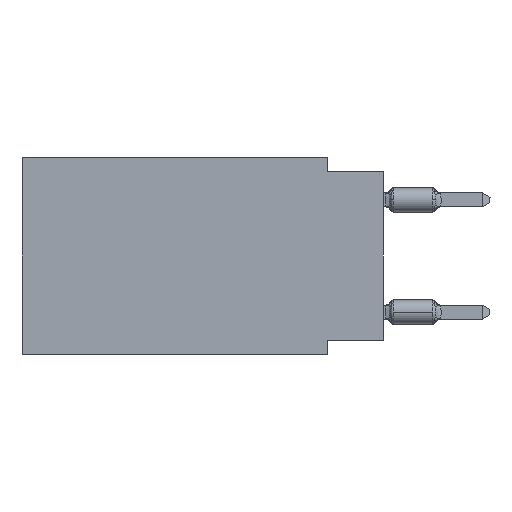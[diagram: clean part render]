
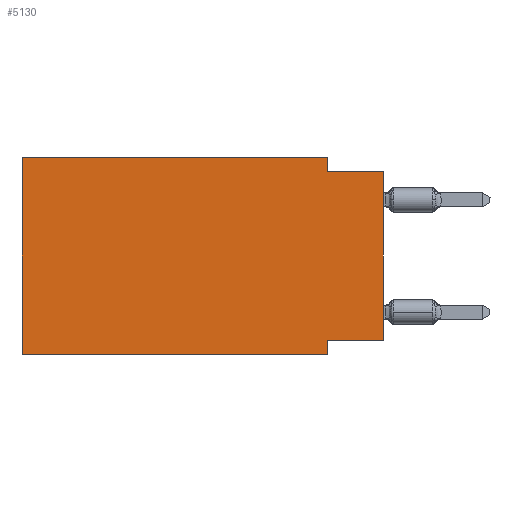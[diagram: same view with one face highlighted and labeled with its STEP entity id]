
A CAD part, left-side view. The second image highlights one B-rep face of the part: STEP entity #5130.
In plain terms, the highlighted planar face has unit normal (-1, 0, 0).
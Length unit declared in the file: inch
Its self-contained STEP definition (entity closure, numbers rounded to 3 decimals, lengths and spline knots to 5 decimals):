
#238 = FACE_OUTER_BOUND ( 'NONE', #5628, .T. ) ;
#494 = EDGE_CURVE ( 'NONE', #7203, #19981, #16778, .T. ) ;
#548 = CARTESIAN_POINT ( 'NONE',  ( 0., 0.1, 0. ) ) ;
#1254 = CARTESIAN_POINT ( 'NONE',  ( 0., 0.645, -0.35 ) ) ;
#1379 = DIRECTION ( 'NONE',  ( 0., 1., 0. ) ) ;
#1858 = VERTEX_POINT ( 'NONE', #18790 ) ;
#2141 = CARTESIAN_POINT ( 'NONE',  ( 0., 0.645, 0. ) ) ;
#2341 = CARTESIAN_POINT ( 'NONE',  ( 0., 0.645, 0. ) ) ;
#2433 = VECTOR ( 'NONE', #20019, 39.37008 ) ;
#2448 = DIRECTION ( 'NONE',  ( 0., 0., -1. ) ) ;
#2746 = ORIENTED_EDGE ( 'NONE', *, *, #9688, .F. ) ;
#2854 = ORIENTED_EDGE ( 'NONE', *, *, #494, .F. ) ;
#2985 = DIRECTION ( 'NONE',  ( 0., 0., 1. ) ) ;
#3105 = VECTOR ( 'NONE', #1379, 39.37008 ) ;
#3199 = CARTESIAN_POINT ( 'NONE',  ( 0., 0.1, 0. ) ) ;
#3248 = EDGE_CURVE ( 'NONE', #12494, #15542, #15832, .T. ) ;
#3467 = DIRECTION ( 'NONE',  ( 0., -1., 0. ) ) ;
#3724 = LINE ( 'NONE', #17938, #3967 ) ;
#3967 = VECTOR ( 'NONE', #10940, 39.37008 ) ;
#4359 = ORIENTED_EDGE ( 'NONE', *, *, #14546, .F. ) ;
#4370 = AXIS2_PLACEMENT_3D ( 'NONE', #2141, #13735, #4744 ) ;
#4707 = LINE ( 'NONE', #1254, #9215 ) ;
#4744 = DIRECTION ( 'NONE',  ( 0., 0., -1. ) ) ;
#5130 = ADVANCED_FACE ( 'NONE', ( #238 ), #7467, .F. ) ;
#5628 = EDGE_LOOP ( 'NONE', ( #13973, #2746, #4359, #2854, #11759, #16143, #15097, #22408 ) ) ;
#6991 = VECTOR ( 'NONE', #3467, 39.37008 ) ;
#7203 = VERTEX_POINT ( 'NONE', #9649 ) ;
#7467 = PLANE ( 'NONE',  #4370 ) ;
#8067 = CARTESIAN_POINT ( 'NONE',  ( 0., 0.1, -0.025 ) ) ;
#8719 = CARTESIAN_POINT ( 'NONE',  ( 0., 0., -0.325 ) ) ;
#9215 = VECTOR ( 'NONE', #11919, 39.37008 ) ;
#9543 = CARTESIAN_POINT ( 'NONE',  ( 0., 0.1, -0.325 ) ) ;
#9649 = CARTESIAN_POINT ( 'NONE',  ( 0., 0.645, 0. ) ) ;
#9688 = EDGE_CURVE ( 'NONE', #15336, #1858, #20151, .T. ) ;
#9895 = DIRECTION ( 'NONE',  ( 0., -1., 0. ) ) ;
#9945 = EDGE_CURVE ( 'NONE', #12494, #1858, #3724, .T. ) ;
#10415 = EDGE_CURVE ( 'NONE', #13206, #20286, #4707, .T. ) ;
#10898 = CARTESIAN_POINT ( 'NONE',  ( 0., 0.1, -0.35 ) ) ;
#10940 = DIRECTION ( 'NONE',  ( 0., 0., 1. ) ) ;
#11204 = EDGE_CURVE ( 'NONE', #13206, #7203, #16962, .T. ) ;
#11492 = EDGE_CURVE ( 'NONE', #15542, #20286, #12795, .T. ) ;
#11759 = ORIENTED_EDGE ( 'NONE', *, *, #11204, .F. ) ;
#11919 = DIRECTION ( 'NONE',  ( 0., -1., 0. ) ) ;
#12494 = VERTEX_POINT ( 'NONE', #17132 ) ;
#12795 = LINE ( 'NONE', #10898, #2433 ) ;
#13206 = VERTEX_POINT ( 'NONE', #13961 ) ;
#13318 = VECTOR ( 'NONE', #2448, 39.37008 ) ;
#13402 = CARTESIAN_POINT ( 'NONE',  ( 0., 0.645, 0. ) ) ;
#13735 = DIRECTION ( 'NONE',  ( 1., 0., 0. ) ) ;
#13764 = VECTOR ( 'NONE', #2985, 39.37008 ) ;
#13961 = CARTESIAN_POINT ( 'NONE',  ( 0., 0.645, -0.35 ) ) ;
#13973 = ORIENTED_EDGE ( 'NONE', *, *, #9945, .T. ) ;
#14546 = EDGE_CURVE ( 'NONE', #19981, #15336, #16775, .T. ) ;
#15097 = ORIENTED_EDGE ( 'NONE', *, *, #11492, .F. ) ;
#15336 = VERTEX_POINT ( 'NONE', #8067 ) ;
#15542 = VERTEX_POINT ( 'NONE', #9543 ) ;
#15832 = LINE ( 'NONE', #8719, #3105 ) ;
#16143 = ORIENTED_EDGE ( 'NONE', *, *, #10415, .T. ) ;
#16775 = LINE ( 'NONE', #548, #13318 ) ;
#16778 = LINE ( 'NONE', #2341, #21627 ) ;
#16962 = LINE ( 'NONE', #13402, #13764 ) ;
#17132 = CARTESIAN_POINT ( 'NONE',  ( 0., 0., -0.325 ) ) ;
#17387 = CARTESIAN_POINT ( 'NONE',  ( 0., 0.1, -0.35 ) ) ;
#17938 = CARTESIAN_POINT ( 'NONE',  ( 0., 0., 0. ) ) ;
#18790 = CARTESIAN_POINT ( 'NONE',  ( 0., 0., -0.025 ) ) ;
#19681 = CARTESIAN_POINT ( 'NONE',  ( 0., 0., -0.025 ) ) ;
#19981 = VERTEX_POINT ( 'NONE', #3199 ) ;
#20019 = DIRECTION ( 'NONE',  ( 0., 0., -1. ) ) ;
#20151 = LINE ( 'NONE', #19681, #6991 ) ;
#20286 = VERTEX_POINT ( 'NONE', #17387 ) ;
#21627 = VECTOR ( 'NONE', #9895, 39.37008 ) ;
#22408 = ORIENTED_EDGE ( 'NONE', *, *, #3248, .F. ) ;
